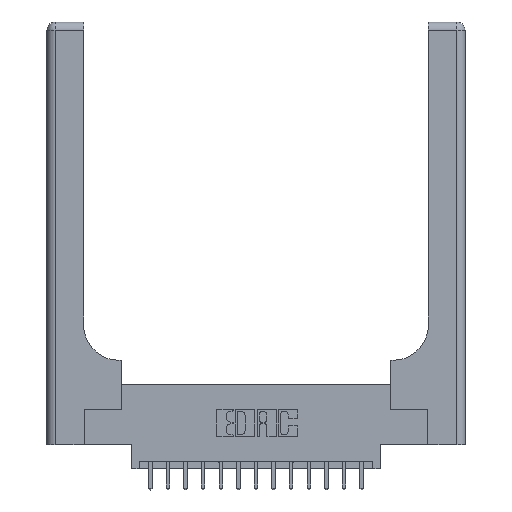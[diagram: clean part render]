
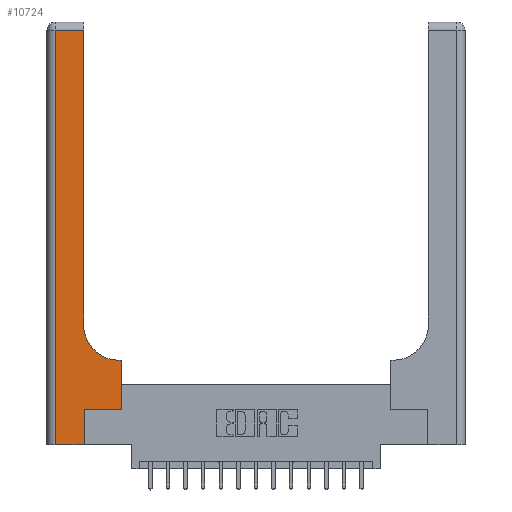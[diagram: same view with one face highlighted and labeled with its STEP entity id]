
A CAD part, top view. The second image highlights one B-rep face of the part: STEP entity #10724.
In plain terms, the highlighted planar face has unit normal (0, 0, 1).
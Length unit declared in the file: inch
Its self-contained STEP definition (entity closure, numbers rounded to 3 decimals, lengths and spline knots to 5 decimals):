
#66 = EDGE_CURVE ( 'NONE', #5664, #14503, #1541, .T. ) ;
#169 = DIRECTION ( 'NONE',  ( 1., 0., 0. ) ) ;
#392 = VECTOR ( 'NONE', #14875, 39.37008 ) ;
#735 = CARTESIAN_POINT ( 'NONE',  ( 0.528, 0.25, 0.37 ) ) ;
#775 = ORIENTED_EDGE ( 'NONE', *, *, #15515, .T. ) ;
#1193 = ORIENTED_EDGE ( 'NONE', *, *, #1454, .T. ) ;
#1224 = DIRECTION ( 'NONE',  ( 0., 0., -1. ) ) ;
#1454 = EDGE_CURVE ( 'NONE', #7925, #2711, #14616, .T. ) ;
#1541 = LINE ( 'NONE', #6977, #8891 ) ;
#1630 = EDGE_CURVE ( 'NONE', #14503, #16349, #13406, .T. ) ;
#1661 = VECTOR ( 'NONE', #16894, 39.37008 ) ;
#1677 = VECTOR ( 'NONE', #4952, 39.37008 ) ;
#1996 = CARTESIAN_POINT ( 'NONE',  ( 0., 2.94, 0.37 ) ) ;
#1997 = ORIENTED_EDGE ( 'NONE', *, *, #8656, .T. ) ;
#2711 = VERTEX_POINT ( 'NONE', #9380 ) ;
#2788 = LINE ( 'NONE', #11293, #9725 ) ;
#3566 = CARTESIAN_POINT ( 'NONE',  ( 0.265, 0.25, 0.37 ) ) ;
#3612 = CARTESIAN_POINT ( 'NONE',  ( 0.51, 0.6, 0.37 ) ) ;
#3630 = VECTOR ( 'NONE', #10407, 39.37008 ) ;
#3866 = EDGE_CURVE ( 'NONE', #14672, #7925, #4892, .T. ) ;
#3881 = ORIENTED_EDGE ( 'NONE', *, *, #66, .T. ) ;
#4239 = ORIENTED_EDGE ( 'NONE', *, *, #4654, .T. ) ;
#4454 = VERTEX_POINT ( 'NONE', #3612 ) ;
#4654 = EDGE_CURVE ( 'NONE', #14975, #5763, #11405, .T. ) ;
#4892 = LINE ( 'NONE', #3566, #1677 ) ;
#4952 = DIRECTION ( 'NONE',  ( 1., 0., 0. ) ) ;
#5152 = CIRCLE ( 'NONE', #15991, 0.25 ) ;
#5664 = VERTEX_POINT ( 'NONE', #8817 ) ;
#5763 = VERTEX_POINT ( 'NONE', #17571 ) ;
#5819 = CARTESIAN_POINT ( 'NONE',  ( 0.528, 0.25, 0.37 ) ) ;
#5912 = AXIS2_PLACEMENT_3D ( 'NONE', #16290, #1224, #10870 ) ;
#6654 = CARTESIAN_POINT ( 'NONE',  ( 0.26, 3., 0.37 ) ) ;
#6746 = EDGE_LOOP ( 'NONE', ( #4239, #775, #3881, #10634, #11025, #9597, #1193, #1997, #15181 ) ) ;
#6977 = CARTESIAN_POINT ( 'NONE',  ( 0.06, 3., 0.37 ) ) ;
#7026 = CARTESIAN_POINT ( 'NONE',  ( 0.51, 0.85, 0.37 ) ) ;
#7317 = CARTESIAN_POINT ( 'NONE',  ( 0.26, 0.85, 0.37 ) ) ;
#7925 = VERTEX_POINT ( 'NONE', #5819 ) ;
#8062 = CARTESIAN_POINT ( 'NONE',  ( 0.265, 0.25, 0.37 ) ) ;
#8442 = DIRECTION ( 'NONE',  ( 1., 0., 0. ) ) ;
#8656 = EDGE_CURVE ( 'NONE', #2711, #4454, #9026, .T. ) ;
#8817 = CARTESIAN_POINT ( 'NONE',  ( 0.06, 2.94, 0.37 ) ) ;
#8891 = VECTOR ( 'NONE', #16580, 39.37008 ) ;
#9026 = LINE ( 'NONE', #10121, #1661 ) ;
#9380 = CARTESIAN_POINT ( 'NONE',  ( 0.528, 0.6, 0.37 ) ) ;
#9502 = PLANE ( 'NONE',  #5912 ) ;
#9597 = ORIENTED_EDGE ( 'NONE', *, *, #3866, .T. ) ;
#9725 = VECTOR ( 'NONE', #16647, 39.37008 ) ;
#10121 = CARTESIAN_POINT ( 'NONE',  ( 0.26, 0.6, 0.37 ) ) ;
#10407 = DIRECTION ( 'NONE',  ( 0., 1., 0. ) ) ;
#10437 = CARTESIAN_POINT ( 'NONE',  ( 0.06, 0., 0.37 ) ) ;
#10634 = ORIENTED_EDGE ( 'NONE', *, *, #1630, .T. ) ;
#10724 = ADVANCED_FACE ( 'NONE', ( #11573 ), #9502, .F. ) ;
#10870 = DIRECTION ( 'NONE',  ( -1., 0., 0. ) ) ;
#11025 = ORIENTED_EDGE ( 'NONE', *, *, #13688, .T. ) ;
#11293 = CARTESIAN_POINT ( 'NONE',  ( 0.265, 0., 0.37 ) ) ;
#11405 = LINE ( 'NONE', #6654, #392 ) ;
#11573 = FACE_OUTER_BOUND ( 'NONE', #6746, .T. ) ;
#12128 = VECTOR ( 'NONE', #169, 39.37008 ) ;
#13213 = VECTOR ( 'NONE', #15742, 39.37008 ) ;
#13406 = LINE ( 'NONE', #16613, #12128 ) ;
#13688 = EDGE_CURVE ( 'NONE', #16349, #14672, #2788, .T. ) ;
#14181 = EDGE_CURVE ( 'NONE', #4454, #14975, #5152, .T. ) ;
#14503 = VERTEX_POINT ( 'NONE', #10437 ) ;
#14616 = LINE ( 'NONE', #735, #3630 ) ;
#14672 = VERTEX_POINT ( 'NONE', #8062 ) ;
#14875 = DIRECTION ( 'NONE',  ( 0., 1., 0. ) ) ;
#14975 = VERTEX_POINT ( 'NONE', #7317 ) ;
#15181 = ORIENTED_EDGE ( 'NONE', *, *, #14181, .T. ) ;
#15515 = EDGE_CURVE ( 'NONE', #5763, #5664, #16808, .T. ) ;
#15742 = DIRECTION ( 'NONE',  ( -1., 0., 0. ) ) ;
#15991 = AXIS2_PLACEMENT_3D ( 'NONE', #7026, #16623, #8442 ) ;
#16018 = CARTESIAN_POINT ( 'NONE',  ( 0.265, 0., 0.37 ) ) ;
#16290 = CARTESIAN_POINT ( 'NONE',  ( 0., 3., 0.37 ) ) ;
#16349 = VERTEX_POINT ( 'NONE', #16018 ) ;
#16580 = DIRECTION ( 'NONE',  ( 0., -1., 0. ) ) ;
#16613 = CARTESIAN_POINT ( 'NONE',  ( 0., 0., 0.37 ) ) ;
#16623 = DIRECTION ( 'NONE',  ( 0., 0., -1. ) ) ;
#16647 = DIRECTION ( 'NONE',  ( 0., 1., 0. ) ) ;
#16808 = LINE ( 'NONE', #1996, #13213 ) ;
#16894 = DIRECTION ( 'NONE',  ( -1., 0., 0. ) ) ;
#17571 = CARTESIAN_POINT ( 'NONE',  ( 0.26, 2.94, 0.37 ) ) ;
